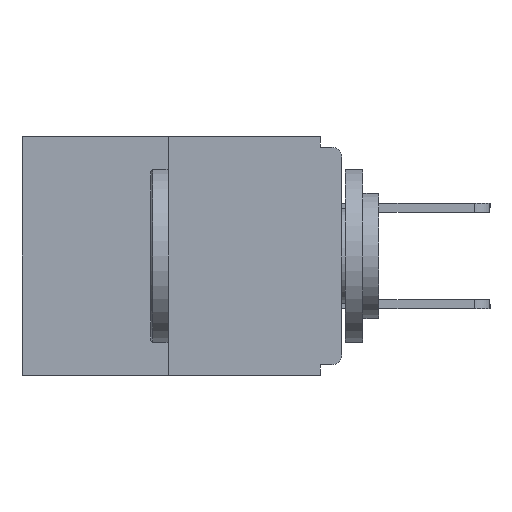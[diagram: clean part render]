
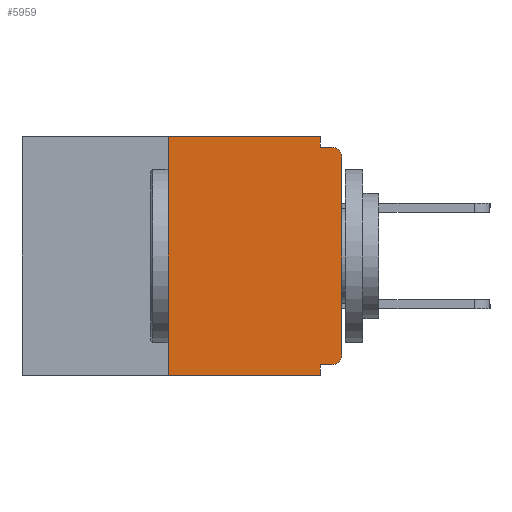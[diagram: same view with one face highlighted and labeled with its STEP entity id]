
A CAD part, left-side view. The second image highlights one B-rep face of the part: STEP entity #5959.
In plain terms, the highlighted planar face has unit normal (-1, 0, 0).
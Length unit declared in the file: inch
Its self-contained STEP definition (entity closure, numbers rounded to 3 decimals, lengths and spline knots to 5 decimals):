
#76 = LINE ( 'NONE', #5691, #3811 ) ;
#323 = ORIENTED_EDGE ( 'NONE', *, *, #12357, .F. ) ;
#325 = CARTESIAN_POINT ( 'NONE',  ( 0., 0.031, -0.328 ) ) ;
#419 = AXIS2_PLACEMENT_3D ( 'NONE', #3539, #4597, #11561 ) ;
#632 = DIRECTION ( 'NONE',  ( 0., 0., -1. ) ) ;
#663 = VECTOR ( 'NONE', #4997, 39.37008 ) ;
#750 = VERTEX_POINT ( 'NONE', #8994 ) ;
#1310 = VERTEX_POINT ( 'NONE', #3057 ) ;
#1341 = DIRECTION ( 'NONE',  ( 0., 1., 0. ) ) ;
#1432 = EDGE_CURVE ( 'NONE', #4393, #5956, #2413, .T. ) ;
#1588 = LINE ( 'NONE', #8314, #1737 ) ;
#1737 = VECTOR ( 'NONE', #8239, 39.37008 ) ;
#2039 = LINE ( 'NONE', #10019, #663 ) ;
#2413 = LINE ( 'NONE', #3275, #2574 ) ;
#2486 = FACE_OUTER_BOUND ( 'NONE', #6038, .T. ) ;
#2574 = VECTOR ( 'NONE', #6223, 39.37008 ) ;
#2855 = ORIENTED_EDGE ( 'NONE', *, *, #3871, .T. ) ;
#2939 = EDGE_CURVE ( 'NONE', #750, #5361, #4569, .T. ) ;
#2952 = CARTESIAN_POINT ( 'NONE',  ( 0., 0.46, -0.343 ) ) ;
#3057 = CARTESIAN_POINT ( 'NONE',  ( 0., 0.031, -0.343 ) ) ;
#3275 = CARTESIAN_POINT ( 'NONE',  ( 0., 0.25, 0. ) ) ;
#3473 = CIRCLE ( 'NONE', #3508, 0.015 ) ;
#3508 = AXIS2_PLACEMENT_3D ( 'NONE', #5708, #9455, #632 ) ;
#3534 = ORIENTED_EDGE ( 'NONE', *, *, #3882, .T. ) ;
#3539 = CARTESIAN_POINT ( 'NONE',  ( 0., 0.015, -0.313 ) ) ;
#3750 = VERTEX_POINT ( 'NONE', #325 ) ;
#3811 = VECTOR ( 'NONE', #5768, 39.37008 ) ;
#3871 = EDGE_CURVE ( 'NONE', #12585, #750, #11644, .T. ) ;
#3882 = EDGE_CURVE ( 'NONE', #5361, #8700, #3473, .T. ) ;
#4393 = VERTEX_POINT ( 'NONE', #4771 ) ;
#4535 = ORIENTED_EDGE ( 'NONE', *, *, #2939, .T. ) ;
#4569 = LINE ( 'NONE', #4681, #7516 ) ;
#4597 = DIRECTION ( 'NONE',  ( -1., 0., 0. ) ) ;
#4681 = CARTESIAN_POINT ( 'NONE',  ( 0., 0., 0. ) ) ;
#4706 = CARTESIAN_POINT ( 'NONE',  ( 0., 0., -0.03 ) ) ;
#4723 = VECTOR ( 'NONE', #5812, 39.37008 ) ;
#4771 = CARTESIAN_POINT ( 'NONE',  ( 0., 0.25, -0.343 ) ) ;
#4997 = DIRECTION ( 'NONE',  ( 0., 0., -1. ) ) ;
#5274 = EDGE_CURVE ( 'NONE', #12585, #3750, #10523, .T. ) ;
#5314 = CARTESIAN_POINT ( 'NONE',  ( 0., 0., -0.015 ) ) ;
#5361 = VERTEX_POINT ( 'NONE', #4706 ) ;
#5395 = VERTEX_POINT ( 'NONE', #12518 ) ;
#5543 = CARTESIAN_POINT ( 'NONE',  ( 0., 0.25, 0. ) ) ;
#5606 = VECTOR ( 'NONE', #1341, 39.37008 ) ;
#5691 = CARTESIAN_POINT ( 'NONE',  ( 0., 0.031, -0.343 ) ) ;
#5708 = CARTESIAN_POINT ( 'NONE',  ( 0., 0.015, -0.03 ) ) ;
#5750 = DIRECTION ( 'NONE',  ( 0., 0., 1. ) ) ;
#5768 = DIRECTION ( 'NONE',  ( 0., 0., -1. ) ) ;
#5812 = DIRECTION ( 'NONE',  ( 0., -1., 0. ) ) ;
#5956 = VERTEX_POINT ( 'NONE', #5543 ) ;
#5959 = ADVANCED_FACE ( 'NONE', ( #2486 ), #11559, .F. ) ;
#6038 = EDGE_LOOP ( 'NONE', ( #323, #12377, #7741, #11587, #10410, #2855, #4535, #3534, #10366, #8920 ) ) ;
#6223 = DIRECTION ( 'NONE',  ( 0., 0., 1. ) ) ;
#6266 = VECTOR ( 'NONE', #12268, 39.37008 ) ;
#6671 = DIRECTION ( 'NONE',  ( 0., 0., -1. ) ) ;
#7516 = VECTOR ( 'NONE', #5750, 39.37008 ) ;
#7541 = DIRECTION ( 'NONE',  ( 1., 0., 0. ) ) ;
#7741 = ORIENTED_EDGE ( 'NONE', *, *, #10698, .T. ) ;
#8239 = DIRECTION ( 'NONE',  ( 0., -1., 0. ) ) ;
#8314 = CARTESIAN_POINT ( 'NONE',  ( 0., 0.46, 0. ) ) ;
#8700 = VERTEX_POINT ( 'NONE', #9387 ) ;
#8815 = EDGE_CURVE ( 'NONE', #3750, #1310, #76, .T. ) ;
#8920 = ORIENTED_EDGE ( 'NONE', *, *, #10969, .F. ) ;
#8994 = CARTESIAN_POINT ( 'NONE',  ( 0., 0., -0.313 ) ) ;
#9387 = CARTESIAN_POINT ( 'NONE',  ( 0., 0.015, -0.015 ) ) ;
#9395 = CARTESIAN_POINT ( 'NONE',  ( 0., 0., -0.328 ) ) ;
#9455 = DIRECTION ( 'NONE',  ( -1., 0., 0. ) ) ;
#10019 = CARTESIAN_POINT ( 'NONE',  ( 0., 0.031, 0. ) ) ;
#10366 = ORIENTED_EDGE ( 'NONE', *, *, #12440, .F. ) ;
#10410 = ORIENTED_EDGE ( 'NONE', *, *, #5274, .F. ) ;
#10523 = LINE ( 'NONE', #9395, #5606 ) ;
#10634 = VERTEX_POINT ( 'NONE', #12591 ) ;
#10665 = CARTESIAN_POINT ( 'NONE',  ( 0., 0.015, -0.328 ) ) ;
#10698 = EDGE_CURVE ( 'NONE', #4393, #1310, #11017, .T. ) ;
#10969 = EDGE_CURVE ( 'NONE', #10634, #5395, #2039, .T. ) ;
#11017 = LINE ( 'NONE', #2952, #4723 ) ;
#11491 = LINE ( 'NONE', #5314, #6266 ) ;
#11559 = PLANE ( 'NONE',  #12331 ) ;
#11561 = DIRECTION ( 'NONE',  ( 0., 0., -1. ) ) ;
#11587 = ORIENTED_EDGE ( 'NONE', *, *, #8815, .F. ) ;
#11644 = CIRCLE ( 'NONE', #419, 0.015 ) ;
#12268 = DIRECTION ( 'NONE',  ( 0., -1., 0. ) ) ;
#12331 = AXIS2_PLACEMENT_3D ( 'NONE', #12530, #7541, #6671 ) ;
#12357 = EDGE_CURVE ( 'NONE', #5956, #10634, #1588, .T. ) ;
#12377 = ORIENTED_EDGE ( 'NONE', *, *, #1432, .F. ) ;
#12440 = EDGE_CURVE ( 'NONE', #5395, #8700, #11491, .T. ) ;
#12518 = CARTESIAN_POINT ( 'NONE',  ( 0., 0.031, -0.015 ) ) ;
#12530 = CARTESIAN_POINT ( 'NONE',  ( 0., 0.46, 0. ) ) ;
#12585 = VERTEX_POINT ( 'NONE', #10665 ) ;
#12591 = CARTESIAN_POINT ( 'NONE',  ( 0., 0.031, 0. ) ) ;
